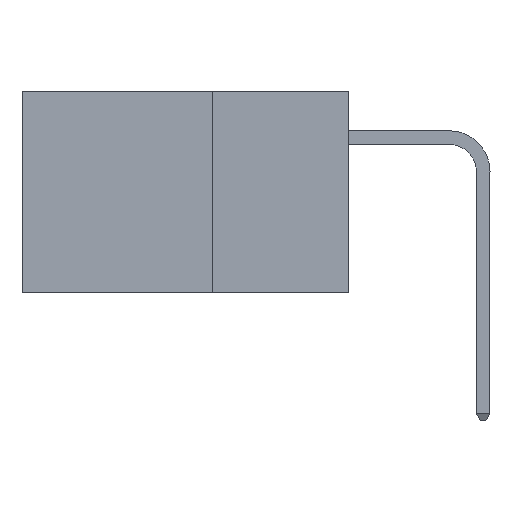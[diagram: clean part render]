
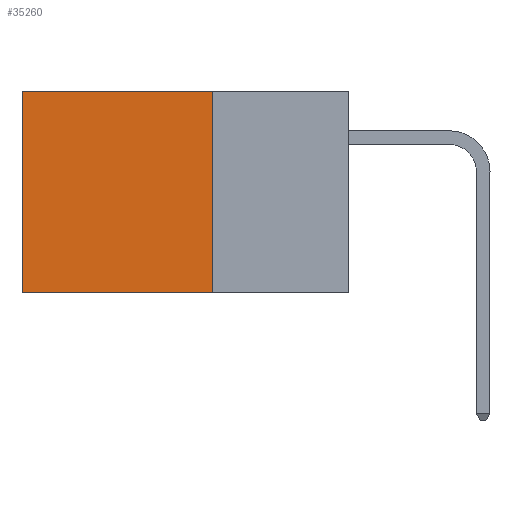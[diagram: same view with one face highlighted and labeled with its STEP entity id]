
A CAD part, left-side view. The second image highlights one B-rep face of the part: STEP entity #35260.
In plain terms, the highlighted planar face has unit normal (-1, 0, 0).
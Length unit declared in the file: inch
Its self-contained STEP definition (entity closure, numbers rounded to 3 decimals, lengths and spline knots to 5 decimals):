
#129 = CARTESIAN_POINT ( 'NONE',  ( 0.2875, 0.25, 0. ) ) ;
#1028 = LINE ( 'NONE', #32461, #5423 ) ;
#1113 = CARTESIAN_POINT ( 'NONE',  ( 0.2875, 0.25, 0. ) ) ;
#2252 = VECTOR ( 'NONE', #21603, 39.37008 ) ;
#5185 = EDGE_CURVE ( 'NONE', #19930, #5656, #26944, .T. ) ;
#5423 = VECTOR ( 'NONE', #24060, 39.37008 ) ;
#5656 = VERTEX_POINT ( 'NONE', #17321 ) ;
#8810 = CARTESIAN_POINT ( 'NONE',  ( 0.2875, 0.25, 0. ) ) ;
#8939 = DIRECTION ( 'NONE',  ( 0., 0., -1. ) ) ;
#9865 = LINE ( 'NONE', #15344, #35054 ) ;
#10724 = ORIENTED_EDGE ( 'NONE', *, *, #34766, .T. ) ;
#11400 = ORIENTED_EDGE ( 'NONE', *, *, #27984, .T. ) ;
#14496 = DIRECTION ( 'NONE',  ( 0., 0., -1. ) ) ;
#15344 = CARTESIAN_POINT ( 'NONE',  ( 0.2875, 0.25, 0. ) ) ;
#16902 = CARTESIAN_POINT ( 'NONE',  ( 0.2875, 0.6, -0.37 ) ) ;
#16908 = FACE_OUTER_BOUND ( 'NONE', #23308, .T. ) ;
#17321 = CARTESIAN_POINT ( 'NONE',  ( 0.2875, 0.25, -0.37 ) ) ;
#18718 = LINE ( 'NONE', #25860, #29290 ) ;
#19930 = VERTEX_POINT ( 'NONE', #129 ) ;
#21319 = AXIS2_PLACEMENT_3D ( 'NONE', #8810, #22851, #8939 ) ;
#21603 = DIRECTION ( 'NONE',  ( 0., 0., -1. ) ) ;
#22851 = DIRECTION ( 'NONE',  ( 1., 0., 0. ) ) ;
#22908 = VERTEX_POINT ( 'NONE', #16902 ) ;
#23308 = EDGE_LOOP ( 'NONE', ( #10724, #26403, #28532, #11400 ) ) ;
#23611 = DIRECTION ( 'NONE',  ( 0., 1., 0. ) ) ;
#24060 = DIRECTION ( 'NONE',  ( 0., 1., 0. ) ) ;
#25860 = CARTESIAN_POINT ( 'NONE',  ( 0.2875, 0.6, 0. ) ) ;
#26403 = ORIENTED_EDGE ( 'NONE', *, *, #36455, .F. ) ;
#26944 = LINE ( 'NONE', #1113, #2252 ) ;
#27984 = EDGE_CURVE ( 'NONE', #19930, #30837, #9865, .T. ) ;
#28532 = ORIENTED_EDGE ( 'NONE', *, *, #5185, .F. ) ;
#28538 = CARTESIAN_POINT ( 'NONE',  ( 0.2875, 0.6, 0. ) ) ;
#29009 = PLANE ( 'NONE',  #21319 ) ;
#29290 = VECTOR ( 'NONE', #14496, 39.37008 ) ;
#30837 = VERTEX_POINT ( 'NONE', #28538 ) ;
#32461 = CARTESIAN_POINT ( 'NONE',  ( 0.2875, 0.25, -0.37 ) ) ;
#34766 = EDGE_CURVE ( 'NONE', #30837, #22908, #18718, .T. ) ;
#35054 = VECTOR ( 'NONE', #23611, 39.37008 ) ;
#35260 = ADVANCED_FACE ( 'NONE', ( #16908 ), #29009, .F. ) ;
#36455 = EDGE_CURVE ( 'NONE', #5656, #22908, #1028, .T. ) ;
